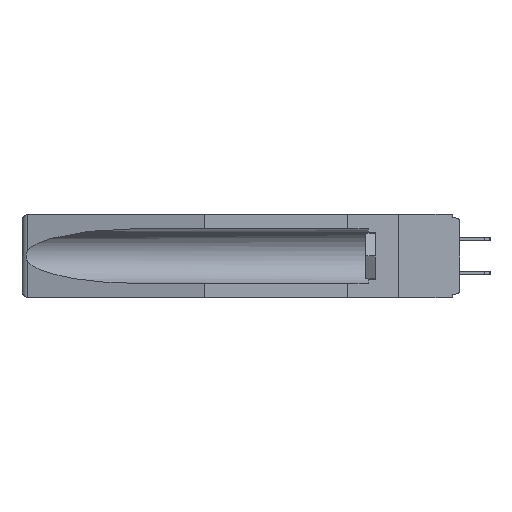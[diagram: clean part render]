
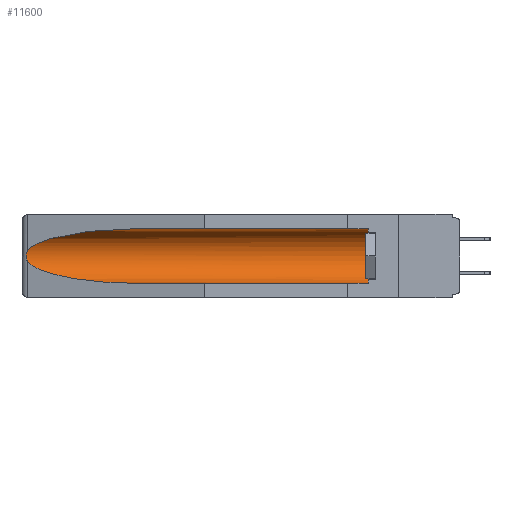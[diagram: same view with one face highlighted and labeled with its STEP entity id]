
A CAD part, left-side view. The second image highlights one B-rep face of the part: STEP entity #11600.
In plain terms, the highlighted cylindrical face has radius 2.857 mm (diameter 5.715 mm), a partial arc.
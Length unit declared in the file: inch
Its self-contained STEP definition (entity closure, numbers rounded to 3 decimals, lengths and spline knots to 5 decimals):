
#358 = ORIENTED_EDGE ( 'NONE', *, *, #9338, .T. ) ;
#630 = DIRECTION ( 'NONE',  ( 0., 1., 0. ) ) ;
#1010 = CARTESIAN_POINT ( 'NONE',  ( 0.26537, 1.52718, -0.19328 ) ) ;
#1759 = DIRECTION ( 'NONE',  ( 0., 1., 0. ) ) ;
#2717 = CARTESIAN_POINT ( 'NONE',  ( 0.25451, 1.48313, -0.24835 ) ) ;
#2938 = CARTESIAN_POINT ( 'NONE',  ( 0.26654, 1.53092, -0.15636 ) ) ;
#3255 = CARTESIAN_POINT ( 'NONE',  ( 0.26597, 1.52961, -0.15275 ) ) ;
#3380 = CYLINDRICAL_SURFACE ( 'NONE', #11112, 0.1125 ) ;
#3443 = VERTEX_POINT ( 'NONE', #15348 ) ;
#3843 = VERTEX_POINT ( 'NONE', #16868 ) ;
#4761 = CARTESIAN_POINT ( 'NONE',  ( 0.26537, 1.52718, -0.14972 ) ) ;
#4991 = CIRCLE ( 'NONE', #29443, 0.1125 ) ;
#5201 = CARTESIAN_POINT ( 'NONE',  ( 0.2673, 1.5327, -0.16383 ) ) ;
#5500 = DIRECTION ( 'NONE',  ( 0., -1., 0. ) ) ;
#5565 = VERTEX_POINT ( 'NONE', #25498 ) ;
#5628 = VERTEX_POINT ( 'NONE', #21579 ) ;
#5683 = EDGE_CURVE ( 'NONE', #8481, #5565, #9971, .T. ) ;
#5950 = FACE_OUTER_BOUND ( 'NONE', #21522, .T. ) ;
#6851 = DIRECTION ( 'NONE',  ( 0., 1., 0. ) ) ;
#7256 = CARTESIAN_POINT ( 'NONE',  ( 0.21114, 1.30732, -0.284 ) ) ;
#7575 = CARTESIAN_POINT ( 'NONE',  ( 0.26537, 1.52718, -0.19328 ) ) ;
#7878 = CARTESIAN_POINT ( 'NONE',  ( 0.2675, 1.53308, -0.17534 ) ) ;
#8481 = VERTEX_POINT ( 'NONE', #1010 ) ;
#9338 = EDGE_CURVE ( 'NONE', #3443, #5628, #4991, .T. ) ;
#9826 = CARTESIAN_POINT ( 'NONE',  ( 0.26537, 1.52718, -0.19328 ) ) ;
#9971 =( BOUNDED_CURVE ( )  B_SPLINE_CURVE ( 3, ( #9826, #2717, #7256, #11799 ),
 .UNSPECIFIED., .F., .F. ) 
 B_SPLINE_CURVE_WITH_KNOTS ( ( 4, 4 ),
 ( 0.1948, 1.5708 ),
 .UNSPECIFIED. ) 
 CURVE ( )  GEOMETRIC_REPRESENTATION_ITEM ( )  RATIONAL_B_SPLINE_CURVE ( ( 1., 0.848, 0.848, 1. ) ) 
 REPRESENTATION_ITEM ( '' )  );
#10118 = CARTESIAN_POINT ( 'NONE',  ( 0.155, 0.126, -0.1715 ) ) ;
#11112 = AXIS2_PLACEMENT_3D ( 'NONE', #17974, #1759, #29771 ) ;
#11600 = ADVANCED_FACE ( 'NONE', ( #5950 ), #3380, .F. ) ;
#11799 = CARTESIAN_POINT ( 'NONE',  ( 0.155, 1.07973, -0.284 ) ) ;
#13609 =( BOUNDED_CURVE ( )  B_SPLINE_CURVE ( 3, ( #18881, #21536, #19276, #4761 ),
 .UNSPECIFIED., .F., .F. ) 
 B_SPLINE_CURVE_WITH_KNOTS ( ( 4, 4 ),
 ( 4.71239, 6.08839 ),
 .UNSPECIFIED. ) 
 CURVE ( )  GEOMETRIC_REPRESENTATION_ITEM ( )  RATIONAL_B_SPLINE_CURVE ( ( 1., 0.848, 0.848, 1. ) ) 
 REPRESENTATION_ITEM ( '' )  );
#14407 = ORIENTED_EDGE ( 'NONE', *, *, #22666, .T. ) ;
#14441 = CARTESIAN_POINT ( 'NONE',  ( 0.26537, 1.52718, -0.14972 ) ) ;
#14493 = VECTOR ( 'NONE', #6851, 39.37008 ) ;
#14619 = CARTESIAN_POINT ( 'NONE',  ( 0.2675, 1.53308, -0.16763 ) ) ;
#14878 = VERTEX_POINT ( 'NONE', #14441 ) ;
#15348 = CARTESIAN_POINT ( 'NONE',  ( 0.155, 0.126, -0.284 ) ) ;
#15583 = LINE ( 'NONE', #25300, #14493 ) ;
#15971 = ORIENTED_EDGE ( 'NONE', *, *, #24371, .T. ) ;
#16868 = CARTESIAN_POINT ( 'NONE',  ( 0.155, 1.07973, -0.059 ) ) ;
#17974 = CARTESIAN_POINT ( 'NONE',  ( 0.155, -0.30754, -0.1715 ) ) ;
#18881 = CARTESIAN_POINT ( 'NONE',  ( 0.155, 1.07973, -0.059 ) ) ;
#19276 = CARTESIAN_POINT ( 'NONE',  ( 0.25451, 1.48313, -0.09465 ) ) ;
#19545 = EDGE_CURVE ( 'NONE', #3443, #5565, #15583, .T. ) ;
#19741 = CARTESIAN_POINT ( 'NONE',  ( 0.26537, 1.52718, -0.14972 ) ) ;
#19947 = ORIENTED_EDGE ( 'NONE', *, *, #20367, .T. ) ;
#20201 = LINE ( 'NONE', #23697, #27205 ) ;
#20367 = EDGE_CURVE ( 'NONE', #3843, #14878, #13609, .T. ) ;
#21522 = EDGE_LOOP ( 'NONE', ( #19947, #14407, #23808, #27438, #358, #15971 ) ) ;
#21536 = CARTESIAN_POINT ( 'NONE',  ( 0.21114, 1.30732, -0.059 ) ) ;
#21579 = CARTESIAN_POINT ( 'NONE',  ( 0.155, 0.126, -0.059 ) ) ;
#22666 = EDGE_CURVE ( 'NONE', #14878, #8481, #24154, .T. ) ;
#23697 = CARTESIAN_POINT ( 'NONE',  ( 0.155, -0.30754, -0.059 ) ) ;
#23808 = ORIENTED_EDGE ( 'NONE', *, *, #5683, .T. ) ;
#24154 = B_SPLINE_CURVE_WITH_KNOTS ( 'NONE', 3,
 ( #19741, #3255, #2938, #5201, #14619, #7878, #29102, #26634, #26330, #7575 ),
 .UNSPECIFIED., .F., .F.,
 ( 4, 2, 2, 2, 4 ),
 ( 0., 0.00029, 0.00058, 0.00087, 0.00117 ),
 .UNSPECIFIED. ) ;
#24371 = EDGE_CURVE ( 'NONE', #5628, #3843, #20201, .T. ) ;
#25300 = CARTESIAN_POINT ( 'NONE',  ( 0.155, -0.30754, -0.284 ) ) ;
#25498 = CARTESIAN_POINT ( 'NONE',  ( 0.155, 1.07973, -0.284 ) ) ;
#26330 = CARTESIAN_POINT ( 'NONE',  ( 0.26597, 1.5296, -0.19026 ) ) ;
#26617 = DIRECTION ( 'NONE',  ( 0., 0., 1. ) ) ;
#26634 = CARTESIAN_POINT ( 'NONE',  ( 0.26655, 1.53094, -0.18657 ) ) ;
#27205 = VECTOR ( 'NONE', #630, 39.37008 ) ;
#27438 = ORIENTED_EDGE ( 'NONE', *, *, #19545, .F. ) ;
#29102 = CARTESIAN_POINT ( 'NONE',  ( 0.2673, 1.53269, -0.17917 ) ) ;
#29443 = AXIS2_PLACEMENT_3D ( 'NONE', #10118, #5500, #26617 ) ;
#29771 = DIRECTION ( 'NONE',  ( 0., 0., 1. ) ) ;
